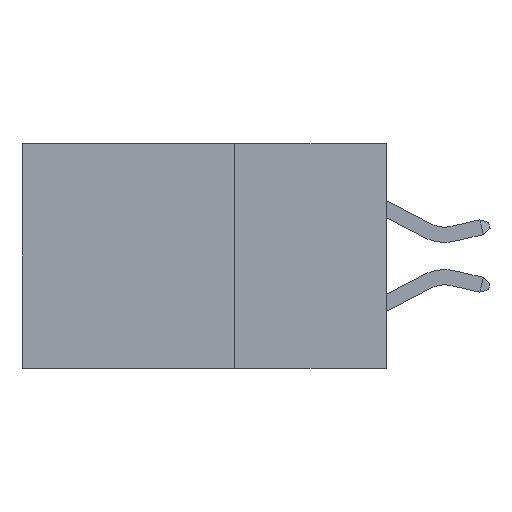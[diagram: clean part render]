
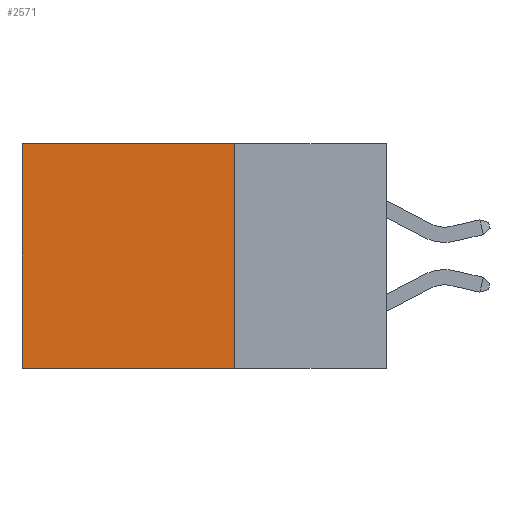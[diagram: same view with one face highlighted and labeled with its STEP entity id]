
A CAD part, left-side view. The second image highlights one B-rep face of the part: STEP entity #2571.
In plain terms, the highlighted planar face has unit normal (-1, 0, 0).
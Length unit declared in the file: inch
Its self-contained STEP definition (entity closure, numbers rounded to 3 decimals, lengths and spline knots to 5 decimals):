
#629 = VECTOR ( 'NONE', #11745, 39.37008 ) ;
#1341 = EDGE_CURVE ( 'NONE', #3021, #2554, #12229, .T. ) ;
#1758 = VERTEX_POINT ( 'NONE', #9253 ) ;
#2554 = VERTEX_POINT ( 'NONE', #16327 ) ;
#2571 = ADVANCED_FACE ( 'NONE', ( #5886 ), #3329, .F. ) ;
#2644 = VERTEX_POINT ( 'NONE', #13983 ) ;
#3021 = VERTEX_POINT ( 'NONE', #9216 ) ;
#3329 = PLANE ( 'NONE',  #4983 ) ;
#4005 = EDGE_CURVE ( 'NONE', #1758, #3021, #10633, .T. ) ;
#4600 = CARTESIAN_POINT ( 'NONE',  ( 0.298, 0.25, 0. ) ) ;
#4983 = AXIS2_PLACEMENT_3D ( 'NONE', #4600, #12793, #7122 ) ;
#5243 = EDGE_LOOP ( 'NONE', ( #16925, #14461, #19521, #13367 ) ) ;
#5886 = FACE_OUTER_BOUND ( 'NONE', #5243, .T. ) ;
#6421 = DIRECTION ( 'NONE',  ( 0., 0., -1. ) ) ;
#7023 = VECTOR ( 'NONE', #13952, 39.37008 ) ;
#7122 = DIRECTION ( 'NONE',  ( 0., 0., -1. ) ) ;
#7557 = DIRECTION ( 'NONE',  ( 0., 1., 0. ) ) ;
#8100 = CARTESIAN_POINT ( 'NONE',  ( 0.298, 0.25, -0.37 ) ) ;
#8330 = EDGE_CURVE ( 'NONE', #2644, #2554, #14503, .T. ) ;
#9216 = CARTESIAN_POINT ( 'NONE',  ( 0.298, 0.25, -0.37 ) ) ;
#9253 = CARTESIAN_POINT ( 'NONE',  ( 0.298, 0.25, 0. ) ) ;
#10232 = CARTESIAN_POINT ( 'NONE',  ( 0.298, 0.25, 0. ) ) ;
#10633 = LINE ( 'NONE', #13925, #7023 ) ;
#11745 = DIRECTION ( 'NONE',  ( 0., 1., 0. ) ) ;
#12229 = LINE ( 'NONE', #8100, #19367 ) ;
#12377 = LINE ( 'NONE', #10232, #629 ) ;
#12793 = DIRECTION ( 'NONE',  ( 1., 0., 0. ) ) ;
#13011 = EDGE_CURVE ( 'NONE', #1758, #2644, #12377, .T. ) ;
#13367 = ORIENTED_EDGE ( 'NONE', *, *, #13011, .T. ) ;
#13925 = CARTESIAN_POINT ( 'NONE',  ( 0.298, 0.25, 0. ) ) ;
#13952 = DIRECTION ( 'NONE',  ( 0., 0., -1. ) ) ;
#13983 = CARTESIAN_POINT ( 'NONE',  ( 0.298, 0.6, 0. ) ) ;
#14461 = ORIENTED_EDGE ( 'NONE', *, *, #1341, .F. ) ;
#14503 = LINE ( 'NONE', #18612, #18096 ) ;
#16327 = CARTESIAN_POINT ( 'NONE',  ( 0.298, 0.6, -0.37 ) ) ;
#16925 = ORIENTED_EDGE ( 'NONE', *, *, #8330, .T. ) ;
#18096 = VECTOR ( 'NONE', #6421, 39.37008 ) ;
#18612 = CARTESIAN_POINT ( 'NONE',  ( 0.298, 0.6, 0. ) ) ;
#19367 = VECTOR ( 'NONE', #7557, 39.37008 ) ;
#19521 = ORIENTED_EDGE ( 'NONE', *, *, #4005, .F. ) ;
